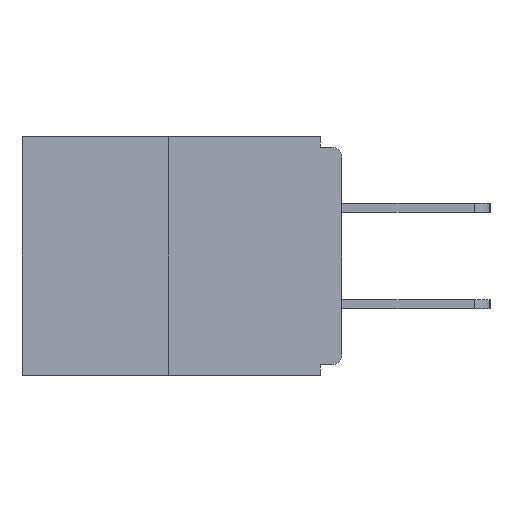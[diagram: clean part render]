
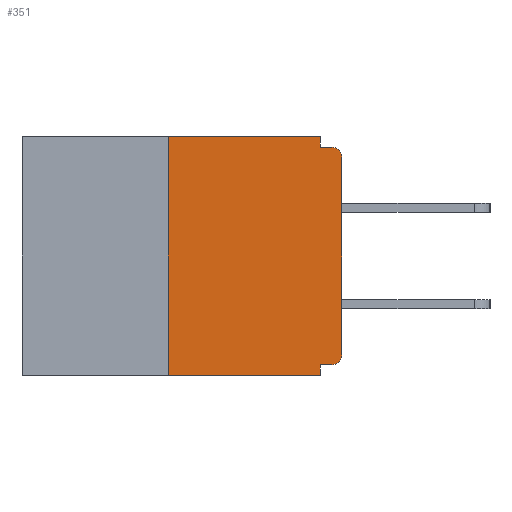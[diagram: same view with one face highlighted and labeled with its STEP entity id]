
A CAD part, left-side view. The second image highlights one B-rep face of the part: STEP entity #351.
In plain terms, the highlighted planar face has unit normal (-1, 0, 0).
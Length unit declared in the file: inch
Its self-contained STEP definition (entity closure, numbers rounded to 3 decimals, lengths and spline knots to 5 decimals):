
#340 = LINE ( 'NONE', #10526, #8734 ) ;
#351 = ADVANCED_FACE ( 'NONE', ( #5356 ), #4557, .F. ) ;
#783 = EDGE_CURVE ( 'NONE', #11329, #6302, #5123, .T. ) ;
#828 = VERTEX_POINT ( 'NONE', #17249 ) ;
#1053 = VERTEX_POINT ( 'NONE', #6402 ) ;
#1261 = ORIENTED_EDGE ( 'NONE', *, *, #783, .T. ) ;
#1803 = CARTESIAN_POINT ( 'NONE',  ( 0., 0.015, -0.328 ) ) ;
#1844 = CARTESIAN_POINT ( 'NONE',  ( 0., 0.031, 0. ) ) ;
#1905 = CARTESIAN_POINT ( 'NONE',  ( 0., 0.46, -0.343 ) ) ;
#2331 = CARTESIAN_POINT ( 'NONE',  ( 0., 0.015, -0.03 ) ) ;
#3290 = DIRECTION ( 'NONE',  ( 0., 1., 0. ) ) ;
#3866 = ORIENTED_EDGE ( 'NONE', *, *, #11547, .F. ) ;
#4339 = DIRECTION ( 'NONE',  ( 0., 0., -1. ) ) ;
#4557 = PLANE ( 'NONE',  #15400 ) ;
#4684 = DIRECTION ( 'NONE',  ( 1., 0., 0. ) ) ;
#4870 = VECTOR ( 'NONE', #7005, 39.37008 ) ;
#4928 = LINE ( 'NONE', #1844, #13082 ) ;
#4966 = VERTEX_POINT ( 'NONE', #12399 ) ;
#5105 = LINE ( 'NONE', #18580, #4870 ) ;
#5123 = CIRCLE ( 'NONE', #10812, 0.015 ) ;
#5279 = EDGE_CURVE ( 'NONE', #828, #1053, #4928, .T. ) ;
#5356 = FACE_OUTER_BOUND ( 'NONE', #9314, .T. ) ;
#5579 = EDGE_CURVE ( 'NONE', #7373, #828, #8945, .T. ) ;
#5677 = CARTESIAN_POINT ( 'NONE',  ( 0., 0.015, -0.015 ) ) ;
#6025 = DIRECTION ( 'NONE',  ( 0., 0., -1. ) ) ;
#6302 = VERTEX_POINT ( 'NONE', #5677 ) ;
#6402 = CARTESIAN_POINT ( 'NONE',  ( 0., 0.031, -0.015 ) ) ;
#6751 = ORIENTED_EDGE ( 'NONE', *, *, #11446, .F. ) ;
#6983 = ORIENTED_EDGE ( 'NONE', *, *, #5579, .F. ) ;
#7005 = DIRECTION ( 'NONE',  ( 0., 0., -1. ) ) ;
#7008 = VERTEX_POINT ( 'NONE', #14791 ) ;
#7081 = VECTOR ( 'NONE', #14865, 39.37008 ) ;
#7373 = VERTEX_POINT ( 'NONE', #11934 ) ;
#7446 = EDGE_CURVE ( 'NONE', #7008, #11329, #14292, .T. ) ;
#7451 = CARTESIAN_POINT ( 'NONE',  ( 0., 0., 0. ) ) ;
#7467 = VERTEX_POINT ( 'NONE', #1803 ) ;
#8110 = VECTOR ( 'NONE', #3290, 39.37008 ) ;
#8264 = CARTESIAN_POINT ( 'NONE',  ( 0., 0.031, -0.328 ) ) ;
#8734 = VECTOR ( 'NONE', #17714, 39.37008 ) ;
#8945 = LINE ( 'NONE', #15939, #16341 ) ;
#9314 = EDGE_LOOP ( 'NONE', ( #6983, #3866, #10451, #18523, #9494, #13549, #18479, #1261, #6751, #14081 ) ) ;
#9494 = ORIENTED_EDGE ( 'NONE', *, *, #11743, .F. ) ;
#9966 = VECTOR ( 'NONE', #17876, 39.37008 ) ;
#10294 = VECTOR ( 'NONE', #10952, 39.37008 ) ;
#10451 = ORIENTED_EDGE ( 'NONE', *, *, #13536, .T. ) ;
#10526 = CARTESIAN_POINT ( 'NONE',  ( 0., 0.25, 0. ) ) ;
#10812 = AXIS2_PLACEMENT_3D ( 'NONE', #2331, #18329, #11031 ) ;
#10952 = DIRECTION ( 'NONE',  ( 0., -1., 0. ) ) ;
#11031 = DIRECTION ( 'NONE',  ( 0., 0., -1. ) ) ;
#11199 = LINE ( 'NONE', #18422, #10294 ) ;
#11329 = VERTEX_POINT ( 'NONE', #13673 ) ;
#11446 = EDGE_CURVE ( 'NONE', #1053, #6302, #11199, .T. ) ;
#11547 = EDGE_CURVE ( 'NONE', #4966, #7373, #340, .T. ) ;
#11713 = CIRCLE ( 'NONE', #18317, 0.015 ) ;
#11743 = EDGE_CURVE ( 'NONE', #7467, #12251, #11939, .T. ) ;
#11795 = CARTESIAN_POINT ( 'NONE',  ( 0., 0.46, 0. ) ) ;
#11934 = CARTESIAN_POINT ( 'NONE',  ( 0., 0.25, 0. ) ) ;
#11939 = LINE ( 'NONE', #15018, #8110 ) ;
#12251 = VERTEX_POINT ( 'NONE', #8264 ) ;
#12399 = CARTESIAN_POINT ( 'NONE',  ( 0., 0.25, -0.343 ) ) ;
#13082 = VECTOR ( 'NONE', #13281, 39.37008 ) ;
#13281 = DIRECTION ( 'NONE',  ( 0., 0., -1. ) ) ;
#13327 = DIRECTION ( 'NONE',  ( 0., -1., 0. ) ) ;
#13536 = EDGE_CURVE ( 'NONE', #4966, #18359, #13807, .T. ) ;
#13549 = ORIENTED_EDGE ( 'NONE', *, *, #14868, .T. ) ;
#13673 = CARTESIAN_POINT ( 'NONE',  ( 0., 0., -0.03 ) ) ;
#13807 = LINE ( 'NONE', #1905, #9966 ) ;
#14081 = ORIENTED_EDGE ( 'NONE', *, *, #5279, .F. ) ;
#14292 = LINE ( 'NONE', #7451, #7081 ) ;
#14558 = CARTESIAN_POINT ( 'NONE',  ( 0., 0.015, -0.313 ) ) ;
#14791 = CARTESIAN_POINT ( 'NONE',  ( 0., 0., -0.313 ) ) ;
#14865 = DIRECTION ( 'NONE',  ( 0., 0., 1. ) ) ;
#14868 = EDGE_CURVE ( 'NONE', #7467, #7008, #11713, .T. ) ;
#15018 = CARTESIAN_POINT ( 'NONE',  ( 0., 0., -0.328 ) ) ;
#15400 = AXIS2_PLACEMENT_3D ( 'NONE', #11795, #4684, #6025 ) ;
#15520 = CARTESIAN_POINT ( 'NONE',  ( 0., 0.031, -0.343 ) ) ;
#15820 = DIRECTION ( 'NONE',  ( -1., 0., 0. ) ) ;
#15939 = CARTESIAN_POINT ( 'NONE',  ( 0., 0.46, 0. ) ) ;
#16186 = EDGE_CURVE ( 'NONE', #12251, #18359, #5105, .T. ) ;
#16341 = VECTOR ( 'NONE', #13327, 39.37008 ) ;
#17249 = CARTESIAN_POINT ( 'NONE',  ( 0., 0.031, 0. ) ) ;
#17714 = DIRECTION ( 'NONE',  ( 0., 0., 1. ) ) ;
#17876 = DIRECTION ( 'NONE',  ( 0., -1., 0. ) ) ;
#18317 = AXIS2_PLACEMENT_3D ( 'NONE', #14558, #15820, #4339 ) ;
#18329 = DIRECTION ( 'NONE',  ( -1., 0., 0. ) ) ;
#18359 = VERTEX_POINT ( 'NONE', #15520 ) ;
#18422 = CARTESIAN_POINT ( 'NONE',  ( 0., 0., -0.015 ) ) ;
#18479 = ORIENTED_EDGE ( 'NONE', *, *, #7446, .T. ) ;
#18523 = ORIENTED_EDGE ( 'NONE', *, *, #16186, .F. ) ;
#18580 = CARTESIAN_POINT ( 'NONE',  ( 0., 0.031, -0.343 ) ) ;
